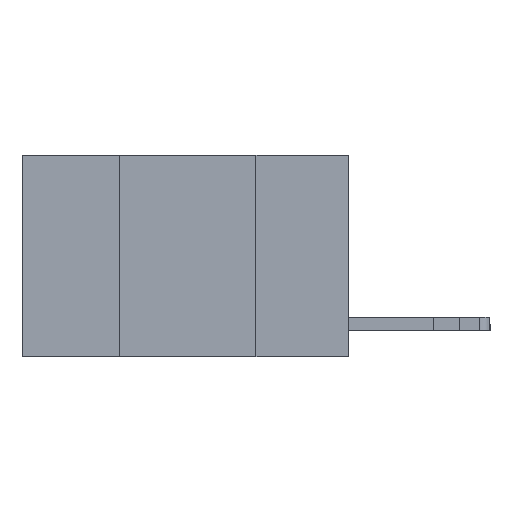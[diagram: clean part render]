
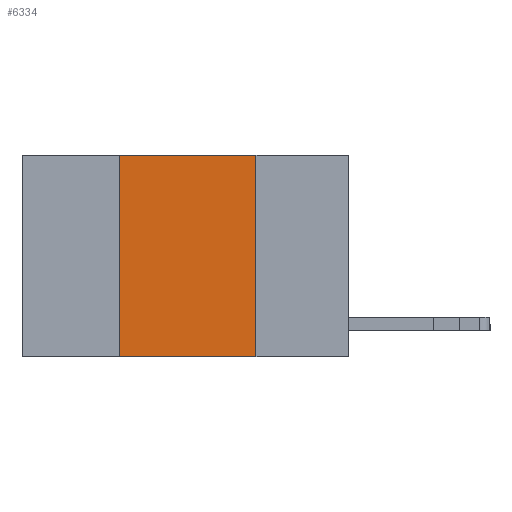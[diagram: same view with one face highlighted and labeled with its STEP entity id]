
A CAD part, left-side view. The second image highlights one B-rep face of the part: STEP entity #6334.
In plain terms, the highlighted planar face has unit normal (-1, 0, 0).
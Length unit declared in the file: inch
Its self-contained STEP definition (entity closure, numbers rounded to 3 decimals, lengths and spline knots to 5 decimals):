
#351 = VERTEX_POINT ( 'NONE', #3535 ) ;
#497 = AXIS2_PLACEMENT_3D ( 'NONE', #10300, #5657, #16655 ) ;
#945 = DIRECTION ( 'NONE',  ( 0., -1., 0. ) ) ;
#1701 = CARTESIAN_POINT ( 'NONE',  ( 0., 0.42, 0. ) ) ;
#3535 = CARTESIAN_POINT ( 'NONE',  ( 0., 0.17, 0. ) ) ;
#3610 = EDGE_LOOP ( 'NONE', ( #10744, #11273, #5421, #19803 ) ) ;
#3651 = VECTOR ( 'NONE', #10421, 39.37008 ) ;
#4033 = EDGE_CURVE ( 'NONE', #8083, #7814, #14365, .T. ) ;
#4615 = EDGE_CURVE ( 'NONE', #8083, #6328, #5575, .T. ) ;
#5124 = DIRECTION ( 'NONE',  ( 0., 0., 1. ) ) ;
#5177 = CARTESIAN_POINT ( 'NONE',  ( 0., 0.42, -0.37 ) ) ;
#5421 = ORIENTED_EDGE ( 'NONE', *, *, #4033, .F. ) ;
#5507 = LINE ( 'NONE', #13496, #19818 ) ;
#5575 = LINE ( 'NONE', #8664, #3651 ) ;
#5657 = DIRECTION ( 'NONE',  ( 1., 0., 0. ) ) ;
#5728 = CARTESIAN_POINT ( 'NONE',  ( 0., 0.6, 0. ) ) ;
#6328 = VERTEX_POINT ( 'NONE', #11978 ) ;
#6334 = ADVANCED_FACE ( 'NONE', ( #12182 ), #7408, .F. ) ;
#6959 = CARTESIAN_POINT ( 'NONE',  ( 0., 0.42, 0. ) ) ;
#7265 = DIRECTION ( 'NONE',  ( 0., 0., -1. ) ) ;
#7408 = PLANE ( 'NONE',  #497 ) ;
#7814 = VERTEX_POINT ( 'NONE', #6959 ) ;
#8083 = VERTEX_POINT ( 'NONE', #5177 ) ;
#8664 = CARTESIAN_POINT ( 'NONE',  ( 0., 0.6, -0.37 ) ) ;
#9009 = EDGE_CURVE ( 'NONE', #351, #6328, #5507, .T. ) ;
#9764 = VECTOR ( 'NONE', #945, 39.37008 ) ;
#10058 = LINE ( 'NONE', #5728, #9764 ) ;
#10300 = CARTESIAN_POINT ( 'NONE',  ( 0., 0.6, 0. ) ) ;
#10421 = DIRECTION ( 'NONE',  ( 0., -1., 0. ) ) ;
#10744 = ORIENTED_EDGE ( 'NONE', *, *, #9009, .F. ) ;
#11273 = ORIENTED_EDGE ( 'NONE', *, *, #19536, .F. ) ;
#11978 = CARTESIAN_POINT ( 'NONE',  ( 0., 0.17, -0.37 ) ) ;
#12182 = FACE_OUTER_BOUND ( 'NONE', #3610, .T. ) ;
#13496 = CARTESIAN_POINT ( 'NONE',  ( 0., 0.17, 0. ) ) ;
#14365 = LINE ( 'NONE', #1701, #20086 ) ;
#16655 = DIRECTION ( 'NONE',  ( 0., 0., -1. ) ) ;
#19536 = EDGE_CURVE ( 'NONE', #7814, #351, #10058, .T. ) ;
#19803 = ORIENTED_EDGE ( 'NONE', *, *, #4615, .T. ) ;
#19818 = VECTOR ( 'NONE', #7265, 39.37008 ) ;
#20086 = VECTOR ( 'NONE', #5124, 39.37008 ) ;
